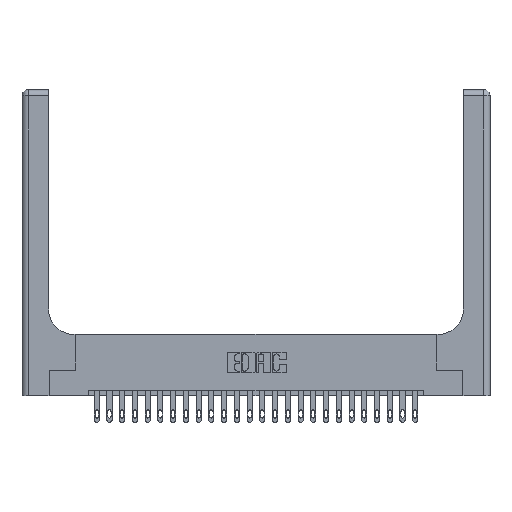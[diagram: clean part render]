
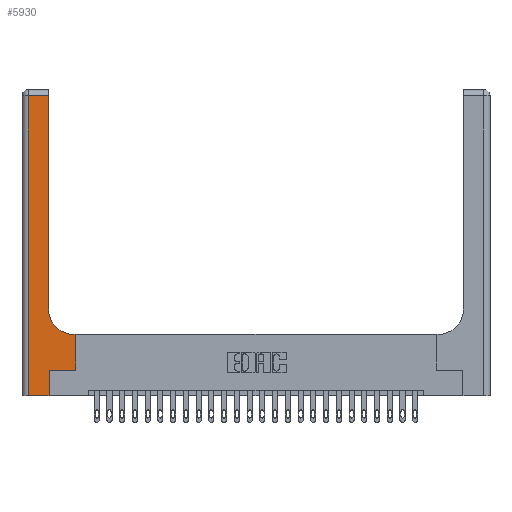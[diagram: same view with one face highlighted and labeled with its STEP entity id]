
A CAD part, top view. The second image highlights one B-rep face of the part: STEP entity #5930.
In plain terms, the highlighted planar face has unit normal (0, 0, 1).
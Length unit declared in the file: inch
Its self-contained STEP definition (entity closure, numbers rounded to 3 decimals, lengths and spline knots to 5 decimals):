
#351 = CARTESIAN_POINT ( 'NONE',  ( 0., 0., 0.37 ) ) ;
#507 = VECTOR ( 'NONE', #19079, 39.37008 ) ;
#660 = CARTESIAN_POINT ( 'NONE',  ( 0.26, 3., 0.37 ) ) ;
#1277 = LINE ( 'NONE', #3027, #17210 ) ;
#1401 = VERTEX_POINT ( 'NONE', #4317 ) ;
#1426 = EDGE_LOOP ( 'NONE', ( #22250, #21420, #9233, #18082, #7570, #5953, #2829, #7876, #16221 ) ) ;
#1442 = CARTESIAN_POINT ( 'NONE',  ( 0.528, 0.6, 0.37 ) ) ;
#1469 = FACE_OUTER_BOUND ( 'NONE', #1426, .T. ) ;
#2354 = LINE ( 'NONE', #21436, #507 ) ;
#2663 = CIRCLE ( 'NONE', #14627, 0.25 ) ;
#2829 = ORIENTED_EDGE ( 'NONE', *, *, #20686, .T. ) ;
#2950 = LINE ( 'NONE', #351, #4449 ) ;
#3027 = CARTESIAN_POINT ( 'NONE',  ( 0.26, 0.6, 0.37 ) ) ;
#3048 = EDGE_CURVE ( 'NONE', #12741, #1401, #2663, .T. ) ;
#3233 = DIRECTION ( 'NONE',  ( 0., 1., 0. ) ) ;
#3617 = EDGE_CURVE ( 'NONE', #22452, #18150, #10366, .T. ) ;
#4317 = CARTESIAN_POINT ( 'NONE',  ( 0.26, 0.85, 0.37 ) ) ;
#4390 = LINE ( 'NONE', #15882, #23589 ) ;
#4449 = VECTOR ( 'NONE', #7995, 39.37008 ) ;
#5466 = LINE ( 'NONE', #20087, #14037 ) ;
#5842 = DIRECTION ( 'NONE',  ( 0., 0., -1. ) ) ;
#5930 = ADVANCED_FACE ( 'NONE', ( #1469 ), #18566, .F. ) ;
#5953 = ORIENTED_EDGE ( 'NONE', *, *, #13223, .T. ) ;
#6210 = VERTEX_POINT ( 'NONE', #1442 ) ;
#6529 = DIRECTION ( 'NONE',  ( 1., 0., 0. ) ) ;
#6783 = CARTESIAN_POINT ( 'NONE',  ( 0.528, 0.25, 0.37 ) ) ;
#6844 = DIRECTION ( 'NONE',  ( -1., 0., 0. ) ) ;
#7155 = DIRECTION ( 'NONE',  ( 0., -1., 0. ) ) ;
#7570 = ORIENTED_EDGE ( 'NONE', *, *, #3617, .T. ) ;
#7876 = ORIENTED_EDGE ( 'NONE', *, *, #13287, .T. ) ;
#7995 = DIRECTION ( 'NONE',  ( 1., 0., 0. ) ) ;
#8247 = VERTEX_POINT ( 'NONE', #20859 ) ;
#8288 = DIRECTION ( 'NONE',  ( 0., 1., 0. ) ) ;
#9233 = ORIENTED_EDGE ( 'NONE', *, *, #12267, .T. ) ;
#9671 = VERTEX_POINT ( 'NONE', #6783 ) ;
#10253 = CARTESIAN_POINT ( 'NONE',  ( 0.265, 0., 0.37 ) ) ;
#10366 = LINE ( 'NONE', #10253, #14190 ) ;
#10572 = CARTESIAN_POINT ( 'NONE',  ( 0.265, 0.25, 0.37 ) ) ;
#11181 = CARTESIAN_POINT ( 'NONE',  ( 0., 3., 0.37 ) ) ;
#11637 = EDGE_CURVE ( 'NONE', #19921, #22452, #2950, .T. ) ;
#12267 = EDGE_CURVE ( 'NONE', #8247, #19921, #24254, .T. ) ;
#12440 = CARTESIAN_POINT ( 'NONE',  ( 0.265, 0., 0.37 ) ) ;
#12741 = VERTEX_POINT ( 'NONE', #14039 ) ;
#12846 = VECTOR ( 'NONE', #8288, 39.37008 ) ;
#13016 = CARTESIAN_POINT ( 'NONE',  ( 0.06, 3., 0.37 ) ) ;
#13223 = EDGE_CURVE ( 'NONE', #18150, #9671, #4390, .T. ) ;
#13283 = VECTOR ( 'NONE', #7155, 39.37008 ) ;
#13287 = EDGE_CURVE ( 'NONE', #6210, #12741, #1277, .T. ) ;
#14037 = VECTOR ( 'NONE', #3233, 39.37008 ) ;
#14039 = CARTESIAN_POINT ( 'NONE',  ( 0.51, 0.6, 0.37 ) ) ;
#14171 = EDGE_CURVE ( 'NONE', #22278, #8247, #2354, .T. ) ;
#14190 = VECTOR ( 'NONE', #17864, 39.37008 ) ;
#14267 = DIRECTION ( 'NONE',  ( -1., 0., 0. ) ) ;
#14627 = AXIS2_PLACEMENT_3D ( 'NONE', #20684, #5842, #17442 ) ;
#15882 = CARTESIAN_POINT ( 'NONE',  ( 0.265, 0.25, 0.37 ) ) ;
#16012 = LINE ( 'NONE', #660, #12846 ) ;
#16221 = ORIENTED_EDGE ( 'NONE', *, *, #3048, .T. ) ;
#16293 = CARTESIAN_POINT ( 'NONE',  ( 0.06, 0., 0.37 ) ) ;
#17210 = VECTOR ( 'NONE', #14267, 39.37008 ) ;
#17442 = DIRECTION ( 'NONE',  ( 1., 0., 0. ) ) ;
#17864 = DIRECTION ( 'NONE',  ( 0., 1., 0. ) ) ;
#18082 = ORIENTED_EDGE ( 'NONE', *, *, #11637, .T. ) ;
#18150 = VERTEX_POINT ( 'NONE', #10572 ) ;
#18566 = PLANE ( 'NONE',  #22662 ) ;
#18799 = DIRECTION ( 'NONE',  ( 0., 0., -1. ) ) ;
#19079 = DIRECTION ( 'NONE',  ( -1., 0., 0. ) ) ;
#19921 = VERTEX_POINT ( 'NONE', #16293 ) ;
#20087 = CARTESIAN_POINT ( 'NONE',  ( 0.528, 0.25, 0.37 ) ) ;
#20315 = EDGE_CURVE ( 'NONE', #1401, #22278, #16012, .T. ) ;
#20684 = CARTESIAN_POINT ( 'NONE',  ( 0.51, 0.85, 0.37 ) ) ;
#20686 = EDGE_CURVE ( 'NONE', #9671, #6210, #5466, .T. ) ;
#20859 = CARTESIAN_POINT ( 'NONE',  ( 0.06, 2.94, 0.37 ) ) ;
#21160 = CARTESIAN_POINT ( 'NONE',  ( 0.26, 2.94, 0.37 ) ) ;
#21420 = ORIENTED_EDGE ( 'NONE', *, *, #14171, .T. ) ;
#21436 = CARTESIAN_POINT ( 'NONE',  ( 0., 2.94, 0.37 ) ) ;
#22250 = ORIENTED_EDGE ( 'NONE', *, *, #20315, .T. ) ;
#22278 = VERTEX_POINT ( 'NONE', #21160 ) ;
#22452 = VERTEX_POINT ( 'NONE', #12440 ) ;
#22662 = AXIS2_PLACEMENT_3D ( 'NONE', #11181, #18799, #6844 ) ;
#23589 = VECTOR ( 'NONE', #6529, 39.37008 ) ;
#24254 = LINE ( 'NONE', #13016, #13283 ) ;
